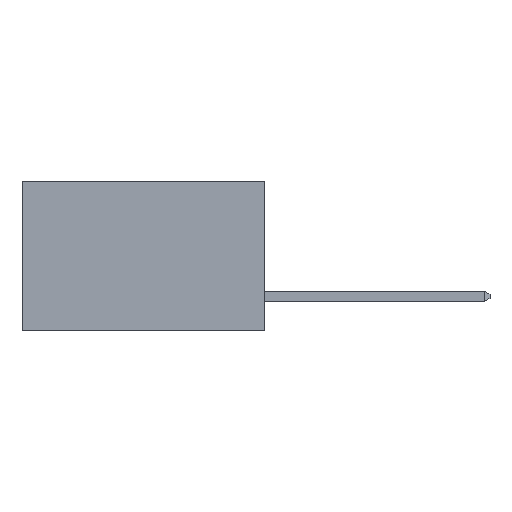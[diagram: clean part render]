
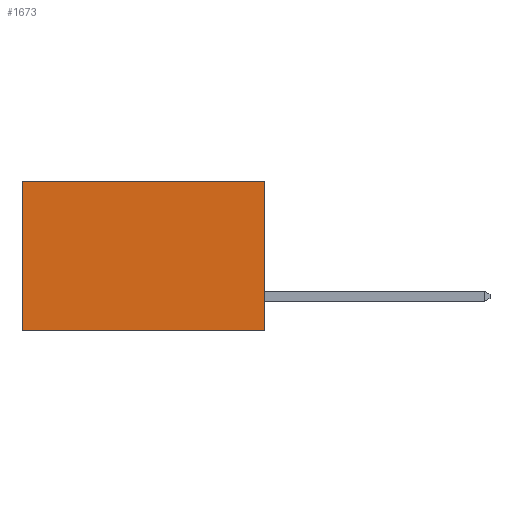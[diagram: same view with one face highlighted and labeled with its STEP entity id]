
A CAD part, left-side view. The second image highlights one B-rep face of the part: STEP entity #1673.
In plain terms, the highlighted planar face has unit normal (-1, 0, 0).
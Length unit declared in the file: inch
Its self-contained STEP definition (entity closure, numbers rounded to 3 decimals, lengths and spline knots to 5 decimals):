
#58 = VECTOR ( 'NONE', #9680, 39.37008 ) ;
#213 = ORIENTED_EDGE ( 'NONE', *, *, #4478, .F. ) ;
#431 = ORIENTED_EDGE ( 'NONE', *, *, #7024, .T. ) ;
#1443 = DIRECTION ( 'NONE',  ( 0., 0., -1. ) ) ;
#1518 = VECTOR ( 'NONE', #5460, 39.37008 ) ;
#1554 = CARTESIAN_POINT ( 'NONE',  ( 0.298, 0., -0.37 ) ) ;
#1673 = ADVANCED_FACE ( 'NONE', ( #10059 ), #2715, .F. ) ;
#2098 = VERTEX_POINT ( 'NONE', #6641 ) ;
#2382 = VERTEX_POINT ( 'NONE', #9230 ) ;
#2715 = PLANE ( 'NONE',  #10772 ) ;
#3052 = DIRECTION ( 'NONE',  ( 0., 0., -1. ) ) ;
#3160 = CARTESIAN_POINT ( 'NONE',  ( 0.298, 0., 0. ) ) ;
#3646 = EDGE_LOOP ( 'NONE', ( #5877, #213, #4868, #431 ) ) ;
#3692 = EDGE_CURVE ( 'NONE', #6266, #2382, #6715, .T. ) ;
#4478 = EDGE_CURVE ( 'NONE', #9339, #2382, #5366, .T. ) ;
#4711 = EDGE_CURVE ( 'NONE', #2098, #9339, #7107, .T. ) ;
#4868 = ORIENTED_EDGE ( 'NONE', *, *, #4711, .F. ) ;
#4917 = CARTESIAN_POINT ( 'NONE',  ( 0.298, 0.6, 0. ) ) ;
#5366 = LINE ( 'NONE', #1554, #58 ) ;
#5460 = DIRECTION ( 'NONE',  ( 0., 0., -1. ) ) ;
#5877 = ORIENTED_EDGE ( 'NONE', *, *, #3692, .T. ) ;
#6266 = VERTEX_POINT ( 'NONE', #10942 ) ;
#6641 = CARTESIAN_POINT ( 'NONE',  ( 0.298, 0., 0. ) ) ;
#6715 = LINE ( 'NONE', #4917, #1518 ) ;
#7024 = EDGE_CURVE ( 'NONE', #2098, #6266, #11567, .T. ) ;
#7107 = LINE ( 'NONE', #8743, #11590 ) ;
#7183 = CARTESIAN_POINT ( 'NONE',  ( 0.298, 0., 0. ) ) ;
#8089 = DIRECTION ( 'NONE',  ( 0., 1., 0. ) ) ;
#8741 = DIRECTION ( 'NONE',  ( 1., 0., 0. ) ) ;
#8743 = CARTESIAN_POINT ( 'NONE',  ( 0.298, 0., 0. ) ) ;
#9230 = CARTESIAN_POINT ( 'NONE',  ( 0.298, 0.6, -0.37 ) ) ;
#9339 = VERTEX_POINT ( 'NONE', #11230 ) ;
#9680 = DIRECTION ( 'NONE',  ( 0., 1., 0. ) ) ;
#10059 = FACE_OUTER_BOUND ( 'NONE', #3646, .T. ) ;
#10772 = AXIS2_PLACEMENT_3D ( 'NONE', #3160, #8741, #3052 ) ;
#10942 = CARTESIAN_POINT ( 'NONE',  ( 0.298, 0.6, 0. ) ) ;
#11230 = CARTESIAN_POINT ( 'NONE',  ( 0.298, 0., -0.37 ) ) ;
#11297 = VECTOR ( 'NONE', #8089, 39.37008 ) ;
#11567 = LINE ( 'NONE', #7183, #11297 ) ;
#11590 = VECTOR ( 'NONE', #1443, 39.37008 ) ;
